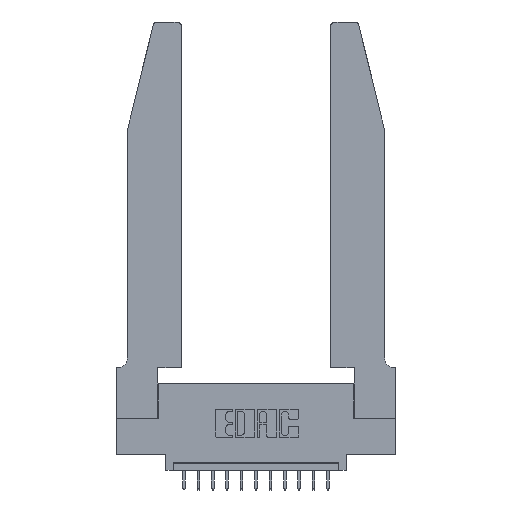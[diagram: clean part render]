
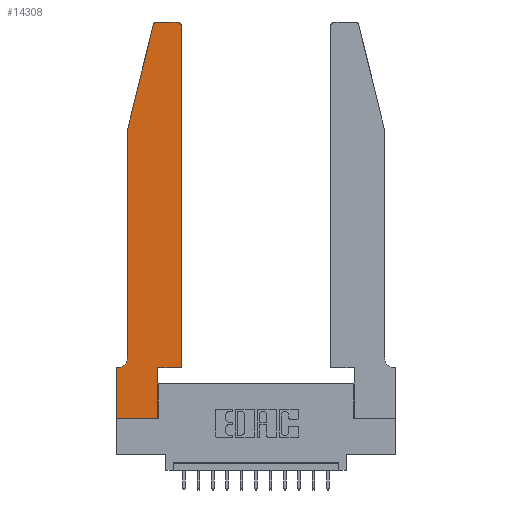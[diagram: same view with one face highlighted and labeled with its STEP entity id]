
A CAD part, top view. The second image highlights one B-rep face of the part: STEP entity #14308.
In plain terms, the highlighted planar face has unit normal (0, 0, 1).
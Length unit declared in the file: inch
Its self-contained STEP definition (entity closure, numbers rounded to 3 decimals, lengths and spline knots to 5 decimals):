
#115 = DIRECTION ( 'NONE',  ( -1., 0., 0. ) ) ;
#179 = ORIENTED_EDGE ( 'NONE', *, *, #12512, .T. ) ;
#701 = PLANE ( 'NONE',  #6421 ) ;
#815 = CARTESIAN_POINT ( 'NONE',  ( 0.2865, 0., 0.37 ) ) ;
#832 = ORIENTED_EDGE ( 'NONE', *, *, #4905, .T. ) ;
#942 = LINE ( 'NONE', #7729, #14103 ) ;
#1087 = VECTOR ( 'NONE', #14258, 39.37008 ) ;
#1633 = CARTESIAN_POINT ( 'NONE',  ( 0., 0., 0.37 ) ) ;
#1718 = VERTEX_POINT ( 'NONE', #8131 ) ;
#1847 = ORIENTED_EDGE ( 'NONE', *, *, #8465, .T. ) ;
#1879 = CARTESIAN_POINT ( 'NONE',  ( 0.0055, 0.42, 0.37 ) ) ;
#1966 = VECTOR ( 'NONE', #16830, 39.37008 ) ;
#2148 = EDGE_CURVE ( 'NONE', #11069, #8057, #7474, .T. ) ;
#2664 = CARTESIAN_POINT ( 'NONE',  ( 0.2605, 2.75, 0.37 ) ) ;
#2695 = CARTESIAN_POINT ( 'NONE',  ( 0.4505, 0.35, 0.37 ) ) ;
#2905 = LINE ( 'NONE', #11130, #3620 ) ;
#3136 = VERTEX_POINT ( 'NONE', #815 ) ;
#3168 = VERTEX_POINT ( 'NONE', #6204 ) ;
#3620 = VECTOR ( 'NONE', #8565, 39.37008 ) ;
#3799 = ORIENTED_EDGE ( 'NONE', *, *, #17038, .T. ) ;
#3926 = DIRECTION ( 'NONE',  ( 0., 0., 1. ) ) ;
#4101 = LINE ( 'NONE', #7021, #6112 ) ;
#4166 = VERTEX_POINT ( 'NONE', #17164 ) ;
#4384 = CARTESIAN_POINT ( 'NONE',  ( 0.0755, 2., 0.37 ) ) ;
#4905 = EDGE_CURVE ( 'NONE', #16717, #4166, #17019, .T. ) ;
#5080 = LINE ( 'NONE', #7709, #1087 ) ;
#5112 = CARTESIAN_POINT ( 'NONE',  ( 0.0055, 0.35, 0.37 ) ) ;
#5498 = EDGE_CURVE ( 'NONE', #13488, #3136, #7107, .T. ) ;
#5878 = CIRCLE ( 'NONE', #11261, 0.03 ) ;
#5957 = ORIENTED_EDGE ( 'NONE', *, *, #16339, .T. ) ;
#6014 = DIRECTION ( 'NONE',  ( 0., 0., -1. ) ) ;
#6019 = ORIENTED_EDGE ( 'NONE', *, *, #13884, .T. ) ;
#6095 = DIRECTION ( 'NONE',  ( 0., 0., 1. ) ) ;
#6112 = VECTOR ( 'NONE', #16366, 39.37008 ) ;
#6204 = CARTESIAN_POINT ( 'NONE',  ( 0.284, 2.75, 0.37 ) ) ;
#6255 = CARTESIAN_POINT ( 'NONE',  ( 0.0755, 0.35, 0.37 ) ) ;
#6343 = EDGE_CURVE ( 'NONE', #10948, #6769, #14047, .T. ) ;
#6421 = AXIS2_PLACEMENT_3D ( 'NONE', #16607, #6095, #8763 ) ;
#6438 = CIRCLE ( 'NONE', #14352, 0.07 ) ;
#6769 = VERTEX_POINT ( 'NONE', #11690 ) ;
#6851 = ORIENTED_EDGE ( 'NONE', *, *, #5498, .T. ) ;
#6872 = EDGE_LOOP ( 'NONE', ( #14427, #7435, #5957, #832, #11161, #7103, #6019, #6851, #3799, #1847, #10690, #179 ) ) ;
#6940 = VECTOR ( 'NONE', #14041, 39.37008 ) ;
#7021 = CARTESIAN_POINT ( 'NONE',  ( 0., 0., 0.37 ) ) ;
#7103 = ORIENTED_EDGE ( 'NONE', *, *, #6343, .T. ) ;
#7107 = LINE ( 'NONE', #1633, #10123 ) ;
#7393 = CARTESIAN_POINT ( 'NONE',  ( 0.4505, 0.35, 0.37 ) ) ;
#7435 = ORIENTED_EDGE ( 'NONE', *, *, #9395, .T. ) ;
#7474 = LINE ( 'NONE', #7393, #6940 ) ;
#7709 = CARTESIAN_POINT ( 'NONE',  ( 0.4505, 0.35, 0.37 ) ) ;
#7729 = CARTESIAN_POINT ( 'NONE',  ( 0.2865, 0.35, 0.37 ) ) ;
#7984 = CARTESIAN_POINT ( 'NONE',  ( 0.4205, 2.72, 0.37 ) ) ;
#8057 = VERTEX_POINT ( 'NONE', #9077 ) ;
#8131 = CARTESIAN_POINT ( 'NONE',  ( 0.4205, 2.75, 0.37 ) ) ;
#8465 = EDGE_CURVE ( 'NONE', #13113, #11069, #5080, .T. ) ;
#8565 = DIRECTION ( 'NONE',  ( -0.239, -0.971, 0. ) ) ;
#8638 = EDGE_CURVE ( 'NONE', #1718, #3168, #14784, .T. ) ;
#8746 = EDGE_CURVE ( 'NONE', #4166, #10948, #6438, .T. ) ;
#8763 = DIRECTION ( 'NONE',  ( 1., 0., 0. ) ) ;
#9077 = CARTESIAN_POINT ( 'NONE',  ( 0.4505, 2.72, 0.37 ) ) ;
#9395 = EDGE_CURVE ( 'NONE', #3168, #14775, #5878, .T. ) ;
#10000 = FACE_OUTER_BOUND ( 'NONE', #6872, .T. ) ;
#10123 = VECTOR ( 'NONE', #15134, 39.37008 ) ;
#10174 = CARTESIAN_POINT ( 'NONE',  ( 0.0755, 2., 0.37 ) ) ;
#10241 = DIRECTION ( 'NONE',  ( 0., -1., 0. ) ) ;
#10690 = ORIENTED_EDGE ( 'NONE', *, *, #2148, .T. ) ;
#10768 = DIRECTION ( 'NONE',  ( 1., 0., 0. ) ) ;
#10835 = CARTESIAN_POINT ( 'NONE',  ( 0., 0., 0.37 ) ) ;
#10948 = VERTEX_POINT ( 'NONE', #5112 ) ;
#11069 = VERTEX_POINT ( 'NONE', #2695 ) ;
#11130 = CARTESIAN_POINT ( 'NONE',  ( 0.0755, 2., 0.37 ) ) ;
#11161 = ORIENTED_EDGE ( 'NONE', *, *, #8746, .T. ) ;
#11261 = AXIS2_PLACEMENT_3D ( 'NONE', #15595, #11470, #10768 ) ;
#11470 = DIRECTION ( 'NONE',  ( 0., 0., 1. ) ) ;
#11690 = CARTESIAN_POINT ( 'NONE',  ( 0., 0.35, 0.37 ) ) ;
#12512 = EDGE_CURVE ( 'NONE', #8057, #1718, #13144, .T. ) ;
#12930 = VECTOR ( 'NONE', #10241, 39.37008 ) ;
#13113 = VERTEX_POINT ( 'NONE', #17098 ) ;
#13134 = DIRECTION ( 'NONE',  ( 0., 1., 0. ) ) ;
#13144 = CIRCLE ( 'NONE', #17337, 0.03 ) ;
#13222 = VECTOR ( 'NONE', #115, 39.37008 ) ;
#13488 = VERTEX_POINT ( 'NONE', #10835 ) ;
#13884 = EDGE_CURVE ( 'NONE', #6769, #13488, #4101, .T. ) ;
#14029 = CARTESIAN_POINT ( 'NONE',  ( 0.25487, 2.72718, 0.37 ) ) ;
#14041 = DIRECTION ( 'NONE',  ( 0., 1., 0. ) ) ;
#14047 = LINE ( 'NONE', #6255, #1966 ) ;
#14103 = VECTOR ( 'NONE', #13134, 39.37008 ) ;
#14258 = DIRECTION ( 'NONE',  ( 1., 0., 0. ) ) ;
#14308 = ADVANCED_FACE ( 'NONE', ( #10000 ), #701, .T. ) ;
#14352 = AXIS2_PLACEMENT_3D ( 'NONE', #1879, #6014, #16518 ) ;
#14427 = ORIENTED_EDGE ( 'NONE', *, *, #8638, .T. ) ;
#14632 = DIRECTION ( 'NONE',  ( 1., 0., 0. ) ) ;
#14775 = VERTEX_POINT ( 'NONE', #14029 ) ;
#14784 = LINE ( 'NONE', #2664, #13222 ) ;
#15134 = DIRECTION ( 'NONE',  ( 1., 0., 0. ) ) ;
#15595 = CARTESIAN_POINT ( 'NONE',  ( 0.284, 2.72, 0.37 ) ) ;
#16339 = EDGE_CURVE ( 'NONE', #14775, #16717, #2905, .T. ) ;
#16366 = DIRECTION ( 'NONE',  ( 0., -1., 0. ) ) ;
#16518 = DIRECTION ( 'NONE',  ( -1., 0., 0. ) ) ;
#16607 = CARTESIAN_POINT ( 'NONE',  ( 0., 0.35, 0.37 ) ) ;
#16717 = VERTEX_POINT ( 'NONE', #4384 ) ;
#16830 = DIRECTION ( 'NONE',  ( -1., 0., 0. ) ) ;
#17019 = LINE ( 'NONE', #10174, #12930 ) ;
#17038 = EDGE_CURVE ( 'NONE', #3136, #13113, #942, .T. ) ;
#17098 = CARTESIAN_POINT ( 'NONE',  ( 0.2865, 0.35, 0.37 ) ) ;
#17164 = CARTESIAN_POINT ( 'NONE',  ( 0.0755, 0.42, 0.37 ) ) ;
#17337 = AXIS2_PLACEMENT_3D ( 'NONE', #7984, #3926, #14632 ) ;
